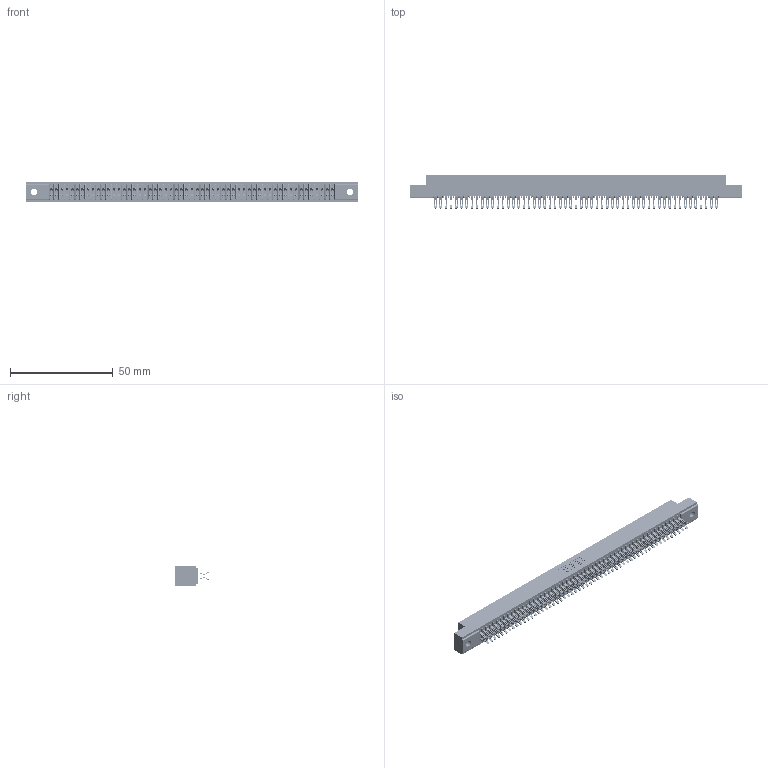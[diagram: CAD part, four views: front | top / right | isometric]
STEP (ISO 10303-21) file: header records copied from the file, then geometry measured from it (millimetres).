
FILE_DESCRIPTION (( 'STEP AP203' ), '1' );
FILE_NAME ('341-110-555-202.STEP', '2018-08-08T12:48:01', ( '' ), ( '' ), 'SwSTEP 2.0', 'SolidWorks 2016', '' );
FILE_SCHEMA (( 'CONFIG_CONTROL_DESIGN' ));
Length unit declared in the file: inch
Products named in the file (3): 341 Part_.128 (3.25) Dia Mounting Holes; 341-292-001_341-292-155; 341-110-555-202
Assembly tree (111 placements, depth 2):
  341-110-555-202
    341 Part_.128 (3.25) Dia Mounting Holes
    341-292-001_341-292-155  x110
Bounding box: 161.93 x 16.31 x 10.16 mm (x, y, z)
Volume: 12068.5 mm3; surface area: 22480.4 mm2
Topology: 111 solids, 111 shells, 8696 faces, 26001 edges, 16926 vertices
Faces by surface type: plane 4688, cylinder 3788, sphere 112, torus 108
Entity records: 65302 total; most frequent: CARTESIAN_POINT 10871, ORIENTED_EDGE 10794, DIRECTION 10531, EDGE_CURVE 5397, LINE 4359, VECTOR 4359, VERTEX_POINT 3410, AXIS2_PLACEMENT_3D 3086
